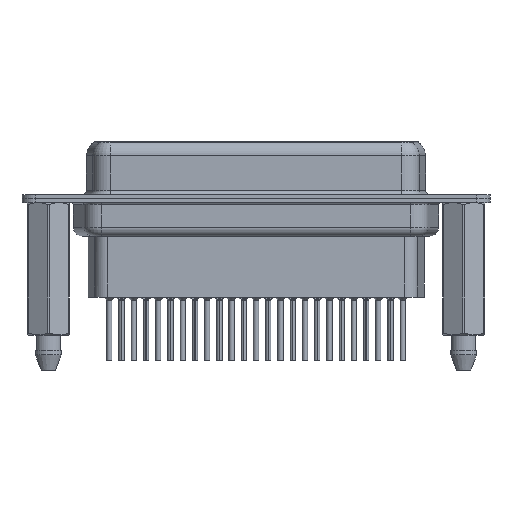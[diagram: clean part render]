
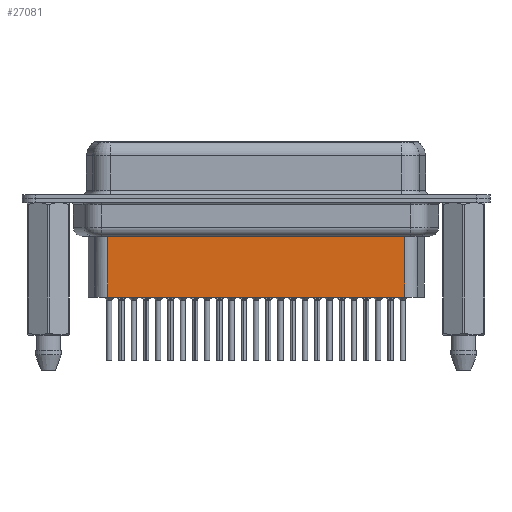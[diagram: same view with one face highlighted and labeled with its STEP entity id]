
A CAD part, front view. The second image highlights one B-rep face of the part: STEP entity #27081.
In plain terms, the highlighted planar face has unit normal (0, -1, 0).
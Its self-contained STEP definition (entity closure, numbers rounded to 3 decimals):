
#219 = EDGE_LOOP ( 'NONE', ( #29112, #2434, #6626, #26267 ) ) ;
#255 = EDGE_CURVE ( 'NONE', #6530, #28672, #12016, .T. ) ;
#881 = VECTOR ( 'NONE', #1076, 1000. ) ;
#1076 = DIRECTION ( 'NONE',  ( -1., 0., 0. ) ) ;
#2434 = ORIENTED_EDGE ( 'NONE', *, *, #255, .T. ) ;
#2628 = EDGE_CURVE ( 'NONE', #22865, #7292, #10015, .T. ) ;
#2919 = DIRECTION ( 'NONE',  ( 0., 0., -1. ) ) ;
#5131 = CARTESIAN_POINT ( 'NONE',  ( 40.344, -3.5, -3.1 ) ) ;
#6530 = VERTEX_POINT ( 'NONE', #17374 ) ;
#6626 = ORIENTED_EDGE ( 'NONE', *, *, #25764, .T. ) ;
#7292 = VERTEX_POINT ( 'NONE', #12035 ) ;
#8112 = DIRECTION ( 'NONE',  ( 1., 0., 0. ) ) ;
#9814 = DIRECTION ( 'NONE',  ( 0., 0., -1. ) ) ;
#10015 = LINE ( 'NONE', #14428, #881 ) ;
#10091 = CARTESIAN_POINT ( 'NONE',  ( 6.706, -3.5, -3.1 ) ) ;
#11713 = EDGE_CURVE ( 'NONE', #6530, #22865, #18359, .T. ) ;
#12016 = LINE ( 'NONE', #18627, #13358 ) ;
#12035 = CARTESIAN_POINT ( 'NONE',  ( 6.706, -3.5, -11.15 ) ) ;
#13315 = CARTESIAN_POINT ( 'NONE',  ( 40.344, -3.5, -11.15 ) ) ;
#13358 = VECTOR ( 'NONE', #16573, 1000. ) ;
#14428 = CARTESIAN_POINT ( 'NONE',  ( 6.706, -3.5, -11.15 ) ) ;
#15925 = FACE_OUTER_BOUND ( 'NONE', #219, .T. ) ;
#16573 = DIRECTION ( 'NONE',  ( -1., 0., 0. ) ) ;
#16856 = LINE ( 'NONE', #10091, #22696 ) ;
#17374 = CARTESIAN_POINT ( 'NONE',  ( 40.344, -3.5, -4.097 ) ) ;
#18359 = LINE ( 'NONE', #5131, #26100 ) ;
#18627 = CARTESIAN_POINT ( 'NONE',  ( 6.459, -3.5, -4.097 ) ) ;
#20052 = PLANE ( 'NONE',  #22758 ) ;
#22696 = VECTOR ( 'NONE', #2919, 1000. ) ;
#22758 = AXIS2_PLACEMENT_3D ( 'NONE', #24942, #28283, #8112 ) ;
#22865 = VERTEX_POINT ( 'NONE', #13315 ) ;
#24098 = CARTESIAN_POINT ( 'NONE',  ( 6.706, -3.5, -4.097 ) ) ;
#24942 = CARTESIAN_POINT ( 'NONE',  ( 6.706, -3.5, -3.1 ) ) ;
#25764 = EDGE_CURVE ( 'NONE', #28672, #7292, #16856, .T. ) ;
#26100 = VECTOR ( 'NONE', #9814, 1000. ) ;
#26267 = ORIENTED_EDGE ( 'NONE', *, *, #2628, .F. ) ;
#27081 = ADVANCED_FACE ( 'NONE', ( #15925 ), #20052, .T. ) ;
#28283 = DIRECTION ( 'NONE',  ( 0., -1., 0. ) ) ;
#28672 = VERTEX_POINT ( 'NONE', #24098 ) ;
#29112 = ORIENTED_EDGE ( 'NONE', *, *, #11713, .F. ) ;
